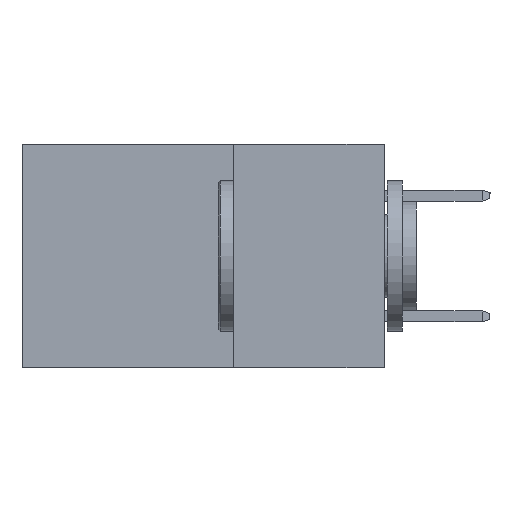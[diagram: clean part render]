
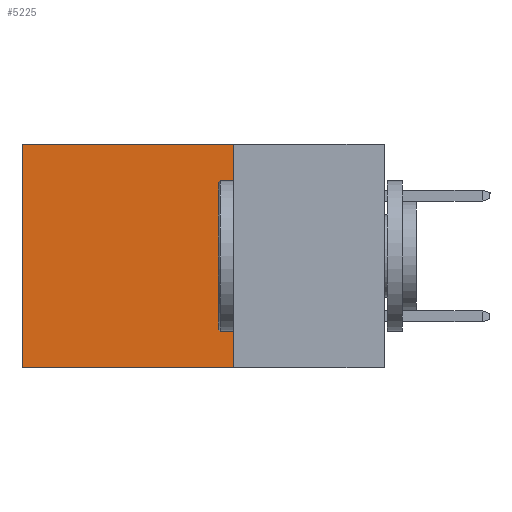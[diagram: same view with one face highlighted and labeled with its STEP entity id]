
A CAD part, left-side view. The second image highlights one B-rep face of the part: STEP entity #5225.
In plain terms, the highlighted planar face has unit normal (-1, 0, 0).
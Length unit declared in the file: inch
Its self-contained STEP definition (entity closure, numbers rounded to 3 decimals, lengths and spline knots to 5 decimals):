
#1517 = CARTESIAN_POINT ( 'NONE',  ( 0.2615, 0.25, -0.37 ) ) ;
#2774 = EDGE_CURVE ( 'NONE', #7081, #10896, #20014, .T. ) ;
#3372 = FACE_OUTER_BOUND ( 'NONE', #12139, .T. ) ;
#4222 = CARTESIAN_POINT ( 'NONE',  ( 0.2615, 0.6, -0.37 ) ) ;
#4622 = ORIENTED_EDGE ( 'NONE', *, *, #7507, .T. ) ;
#5225 = ADVANCED_FACE ( 'NONE', ( #3372 ), #18372, .F. ) ;
#5387 = ORIENTED_EDGE ( 'NONE', *, *, #2774, .F. ) ;
#7081 = VERTEX_POINT ( 'NONE', #7832 ) ;
#7507 = EDGE_CURVE ( 'NONE', #12036, #8084, #15200, .T. ) ;
#7832 = CARTESIAN_POINT ( 'NONE',  ( 0.2615, 0.25, 0. ) ) ;
#8077 = ORIENTED_EDGE ( 'NONE', *, *, #14630, .F. ) ;
#8084 = VERTEX_POINT ( 'NONE', #4222 ) ;
#9845 = VECTOR ( 'NONE', #13168, 39.37008 ) ;
#10023 = DIRECTION ( 'NONE',  ( 0., 0., -1. ) ) ;
#10896 = VERTEX_POINT ( 'NONE', #20089 ) ;
#11798 = CARTESIAN_POINT ( 'NONE',  ( 0.2615, 0.6, 0. ) ) ;
#12036 = VERTEX_POINT ( 'NONE', #11798 ) ;
#12139 = EDGE_LOOP ( 'NONE', ( #4622, #8077, #5387, #18056 ) ) ;
#13168 = DIRECTION ( 'NONE',  ( 0., 1., 0. ) ) ;
#14234 = LINE ( 'NONE', #14349, #15155 ) ;
#14349 = CARTESIAN_POINT ( 'NONE',  ( 0.2615, 0.25, 0. ) ) ;
#14630 = EDGE_CURVE ( 'NONE', #10896, #8084, #21356, .T. ) ;
#14980 = CARTESIAN_POINT ( 'NONE',  ( 0.2615, 0.25, -0.37 ) ) ;
#15155 = VECTOR ( 'NONE', #17391, 39.37008 ) ;
#15200 = LINE ( 'NONE', #17045, #19928 ) ;
#16181 = EDGE_CURVE ( 'NONE', #7081, #12036, #14234, .T. ) ;
#16667 = AXIS2_PLACEMENT_3D ( 'NONE', #14980, #20225, #18265 ) ;
#17045 = CARTESIAN_POINT ( 'NONE',  ( 0.2615, 0.6, -0.37 ) ) ;
#17391 = DIRECTION ( 'NONE',  ( 0., 1., 0. ) ) ;
#18056 = ORIENTED_EDGE ( 'NONE', *, *, #16181, .T. ) ;
#18265 = DIRECTION ( 'NONE',  ( 0., 0., -1. ) ) ;
#18372 = PLANE ( 'NONE',  #16667 ) ;
#18920 = DIRECTION ( 'NONE',  ( 0., 0., -1. ) ) ;
#19184 = VECTOR ( 'NONE', #10023, 39.37008 ) ;
#19513 = CARTESIAN_POINT ( 'NONE',  ( 0.2615, 0.25, -0.37 ) ) ;
#19928 = VECTOR ( 'NONE', #18920, 39.37008 ) ;
#20014 = LINE ( 'NONE', #1517, #19184 ) ;
#20089 = CARTESIAN_POINT ( 'NONE',  ( 0.2615, 0.25, -0.37 ) ) ;
#20225 = DIRECTION ( 'NONE',  ( 1., 0., 0. ) ) ;
#21356 = LINE ( 'NONE', #19513, #9845 ) ;
